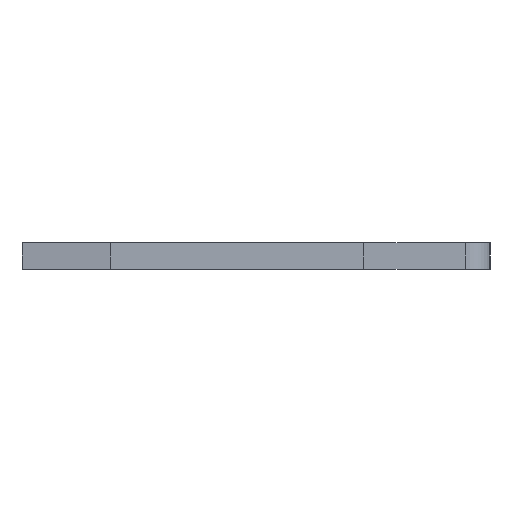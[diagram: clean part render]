
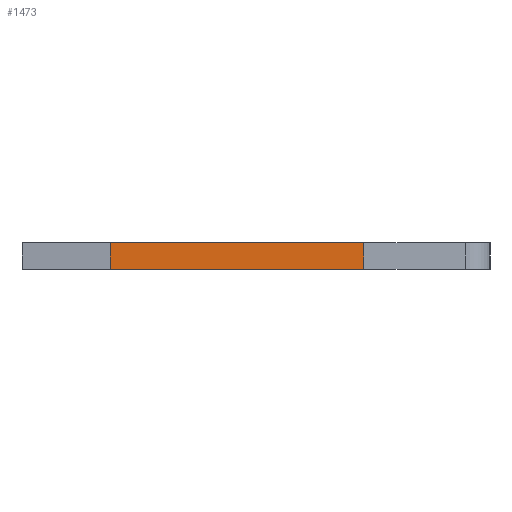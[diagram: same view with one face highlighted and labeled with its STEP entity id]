
A CAD part, left-side view. The second image highlights one B-rep face of the part: STEP entity #1473.
In plain terms, the highlighted face is planar.
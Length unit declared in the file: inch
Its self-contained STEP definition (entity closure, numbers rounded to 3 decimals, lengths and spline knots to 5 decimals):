
#38 = FACE_OUTER_BOUND ( 'NONE', #921, .T. ) ;
#115 = LINE ( 'NONE', #1596, #393 ) ;
#119 = DIRECTION ( 'NONE',  ( 0., 1., 0. ) ) ;
#167 = EDGE_CURVE ( 'NONE', #830, #1601, #1164, .T. ) ;
#175 = DIRECTION ( 'NONE',  ( 0., 1., 0. ) ) ;
#239 = VECTOR ( 'NONE', #285, 39.37008 ) ;
#285 = DIRECTION ( 'NONE',  ( -1., 0., 0. ) ) ;
#317 = CARTESIAN_POINT ( 'NONE',  ( 0.013, 0.146, -0.0575 ) ) ;
#393 = VECTOR ( 'NONE', #175, 39.37008 ) ;
#427 = ORIENTED_EDGE ( 'NONE', *, *, #1016, .T. ) ;
#675 = CARTESIAN_POINT ( 'NONE',  ( 0.013, -0.099, -0.0575 ) ) ;
#784 = DIRECTION ( 'NONE',  ( -1., 0., 0. ) ) ;
#794 = CARTESIAN_POINT ( 'NONE',  ( 0.013, 0.146, -0.0575 ) ) ;
#813 = CARTESIAN_POINT ( 'NONE',  ( 0.013, 0.146, -0.0575 ) ) ;
#830 = VERTEX_POINT ( 'NONE', #1172 ) ;
#921 = EDGE_LOOP ( 'NONE', ( #1067, #1087, #1528, #427 ) ) ;
#976 = DIRECTION ( 'NONE',  ( 0., 0., 1. ) ) ;
#992 = LINE ( 'NONE', #1586, #1531 ) ;
#993 = DIRECTION ( 'NONE',  ( 1., 0., 0. ) ) ;
#1016 = EDGE_CURVE ( 'NONE', #1338, #830, #992, .T. ) ;
#1055 = EDGE_CURVE ( 'NONE', #1192, #1601, #1489, .T. ) ;
#1067 = ORIENTED_EDGE ( 'NONE', *, *, #167, .T. ) ;
#1087 = ORIENTED_EDGE ( 'NONE', *, *, #1055, .F. ) ;
#1109 = PLANE ( 'NONE',  #1341 ) ;
#1164 = LINE ( 'NONE', #1282, #1637 ) ;
#1172 = CARTESIAN_POINT ( 'NONE',  ( -0.013, -0.099, -0.0575 ) ) ;
#1192 = VERTEX_POINT ( 'NONE', #813 ) ;
#1282 = CARTESIAN_POINT ( 'NONE',  ( -0.013, 0.146, -0.0575 ) ) ;
#1309 = EDGE_CURVE ( 'NONE', #1338, #1192, #115, .T. ) ;
#1338 = VERTEX_POINT ( 'NONE', #675 ) ;
#1341 = AXIS2_PLACEMENT_3D ( 'NONE', #317, #976, #993 ) ;
#1473 = ADVANCED_FACE ( 'NONE', ( #38 ), #1109, .F. ) ;
#1489 = LINE ( 'NONE', #794, #239 ) ;
#1524 = CARTESIAN_POINT ( 'NONE',  ( -0.013, 0.146, -0.0575 ) ) ;
#1528 = ORIENTED_EDGE ( 'NONE', *, *, #1309, .F. ) ;
#1531 = VECTOR ( 'NONE', #784, 39.37008 ) ;
#1586 = CARTESIAN_POINT ( 'NONE',  ( 0.013, -0.099, -0.0575 ) ) ;
#1596 = CARTESIAN_POINT ( 'NONE',  ( 0.013, 0.146, -0.0575 ) ) ;
#1601 = VERTEX_POINT ( 'NONE', #1524 ) ;
#1637 = VECTOR ( 'NONE', #119, 39.37008 ) ;
